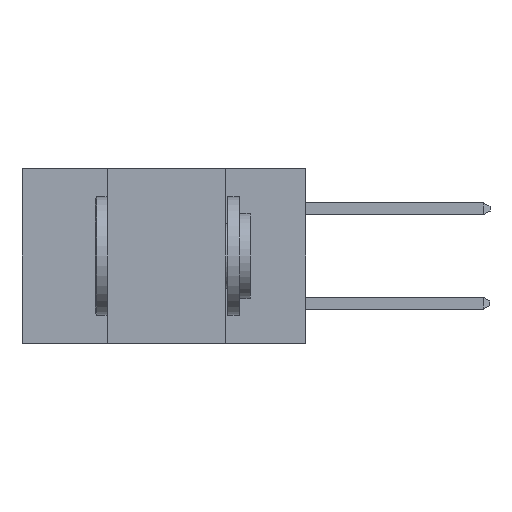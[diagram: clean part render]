
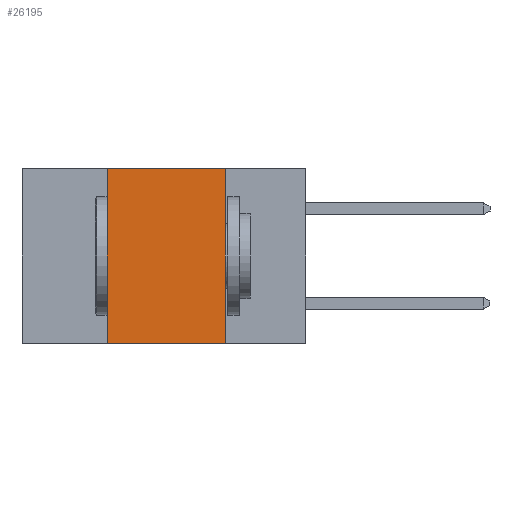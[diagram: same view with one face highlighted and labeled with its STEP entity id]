
A CAD part, left-side view. The second image highlights one B-rep face of the part: STEP entity #26195.
In plain terms, the highlighted planar face has unit normal (-1, 0, 0).
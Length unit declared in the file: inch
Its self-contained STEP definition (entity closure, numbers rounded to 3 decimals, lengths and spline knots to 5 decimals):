
#369 = ORIENTED_EDGE ( 'NONE', *, *, #5698, .F. ) ;
#510 = ORIENTED_EDGE ( 'NONE', *, *, #3439, .F. ) ;
#865 = ORIENTED_EDGE ( 'NONE', *, *, #11026, .F. ) ;
#2012 = ORIENTED_EDGE ( 'NONE', *, *, #17829, .T. ) ;
#2132 = VECTOR ( 'NONE', #8714, 39.37008 ) ;
#2187 = VERTEX_POINT ( 'NONE', #23394 ) ;
#3104 = VECTOR ( 'NONE', #19214, 39.37008 ) ;
#3335 = PLANE ( 'NONE',  #9795 ) ;
#3385 = VERTEX_POINT ( 'NONE', #8294 ) ;
#3439 = EDGE_CURVE ( 'NONE', #14223, #9642, #8177, .T. ) ;
#4510 = CARTESIAN_POINT ( 'NONE',  ( 0., 0.6, 0. ) ) ;
#5618 = DIRECTION ( 'NONE',  ( 0., 0., -1. ) ) ;
#5698 = EDGE_CURVE ( 'NONE', #9642, #3385, #14440, .T. ) ;
#8177 = LINE ( 'NONE', #4510, #2132 ) ;
#8294 = CARTESIAN_POINT ( 'NONE',  ( 0., 0.17, -0.37 ) ) ;
#8714 = DIRECTION ( 'NONE',  ( 0., -1., 0. ) ) ;
#8747 = CARTESIAN_POINT ( 'NONE',  ( 0., 0.17, 0. ) ) ;
#9642 = VERTEX_POINT ( 'NONE', #8747 ) ;
#9795 = AXIS2_PLACEMENT_3D ( 'NONE', #25289, #19061, #5618 ) ;
#11026 = EDGE_CURVE ( 'NONE', #2187, #14223, #20895, .T. ) ;
#14223 = VERTEX_POINT ( 'NONE', #17286 ) ;
#14440 = LINE ( 'NONE', #22717, #3104 ) ;
#17116 = CARTESIAN_POINT ( 'NONE',  ( 0., 0.6, -0.37 ) ) ;
#17286 = CARTESIAN_POINT ( 'NONE',  ( 0., 0.42, 0. ) ) ;
#17829 = EDGE_CURVE ( 'NONE', #2187, #3385, #21983, .T. ) ;
#19061 = DIRECTION ( 'NONE',  ( 1., 0., 0. ) ) ;
#19214 = DIRECTION ( 'NONE',  ( 0., 0., -1. ) ) ;
#19370 = DIRECTION ( 'NONE',  ( 0., -1., 0. ) ) ;
#20895 = LINE ( 'NONE', #24492, #27390 ) ;
#21292 = VECTOR ( 'NONE', #19370, 39.37008 ) ;
#21983 = LINE ( 'NONE', #17116, #21292 ) ;
#22717 = CARTESIAN_POINT ( 'NONE',  ( 0., 0.17, 0. ) ) ;
#23394 = CARTESIAN_POINT ( 'NONE',  ( 0., 0.42, -0.37 ) ) ;
#23513 = EDGE_LOOP ( 'NONE', ( #369, #510, #865, #2012 ) ) ;
#24492 = CARTESIAN_POINT ( 'NONE',  ( 0., 0.42, 0. ) ) ;
#25289 = CARTESIAN_POINT ( 'NONE',  ( 0., 0.6, 0. ) ) ;
#26195 = ADVANCED_FACE ( 'NONE', ( #26605 ), #3335, .F. ) ;
#26605 = FACE_OUTER_BOUND ( 'NONE', #23513, .T. ) ;
#26737 = DIRECTION ( 'NONE',  ( 0., 0., 1. ) ) ;
#27390 = VECTOR ( 'NONE', #26737, 39.37008 ) ;
